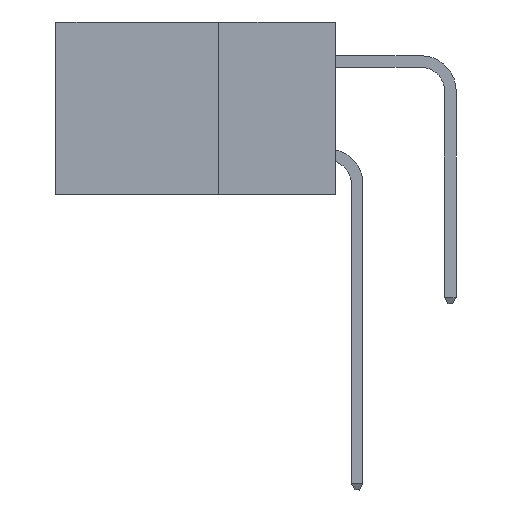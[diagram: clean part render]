
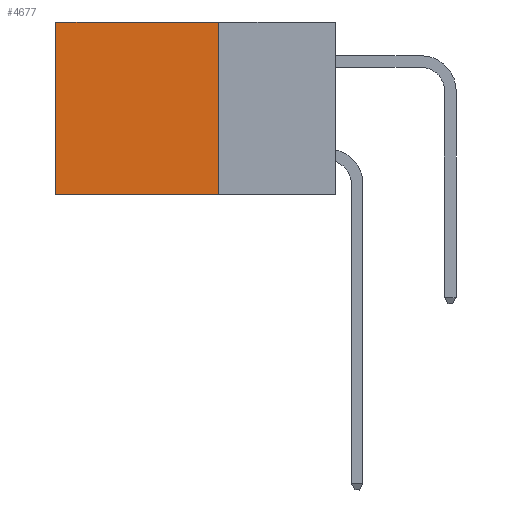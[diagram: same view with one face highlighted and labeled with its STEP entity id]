
A CAD part, left-side view. The second image highlights one B-rep face of the part: STEP entity #4677.
In plain terms, the highlighted planar face has unit normal (-1, 0, 0).
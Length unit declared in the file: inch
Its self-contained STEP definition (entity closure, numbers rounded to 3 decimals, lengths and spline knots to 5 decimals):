
#65 = DIRECTION ( 'NONE',  ( 0., 0., -1. ) ) ;
#344 = LINE ( 'NONE', #15553, #16745 ) ;
#582 = EDGE_CURVE ( 'NONE', #10924, #9720, #9602, .T. ) ;
#599 = CARTESIAN_POINT ( 'NONE',  ( 0.2875, 0.25, 0. ) ) ;
#3356 = PLANE ( 'NONE',  #12624 ) ;
#4250 = DIRECTION ( 'NONE',  ( 0., 1., 0. ) ) ;
#4677 = ADVANCED_FACE ( 'NONE', ( #23413 ), #3356, .F. ) ;
#7243 = CARTESIAN_POINT ( 'NONE',  ( 0.2875, 0.25, -0.37 ) ) ;
#8731 = DIRECTION ( 'NONE',  ( 1., 0., 0. ) ) ;
#8869 = ORIENTED_EDGE ( 'NONE', *, *, #22760, .F. ) ;
#9602 = LINE ( 'NONE', #15096, #15773 ) ;
#9717 = DIRECTION ( 'NONE',  ( 0., 1., 0. ) ) ;
#9720 = VERTEX_POINT ( 'NONE', #10195 ) ;
#10028 = ORIENTED_EDGE ( 'NONE', *, *, #582, .T. ) ;
#10195 = CARTESIAN_POINT ( 'NONE',  ( 0.2875, 0.6, 0. ) ) ;
#10525 = ORIENTED_EDGE ( 'NONE', *, *, #12679, .F. ) ;
#10576 = ORIENTED_EDGE ( 'NONE', *, *, #15108, .T. ) ;
#10594 = VECTOR ( 'NONE', #65, 39.37008 ) ;
#10787 = CARTESIAN_POINT ( 'NONE',  ( 0.2875, 0.25, 0. ) ) ;
#10924 = VERTEX_POINT ( 'NONE', #20815 ) ;
#11332 = DIRECTION ( 'NONE',  ( 0., 0., -1. ) ) ;
#12624 = AXIS2_PLACEMENT_3D ( 'NONE', #10787, #8731, #21712 ) ;
#12679 = EDGE_CURVE ( 'NONE', #10924, #15038, #20909, .T. ) ;
#13196 = CARTESIAN_POINT ( 'NONE',  ( 0.2875, 0.6, 0. ) ) ;
#13435 = LINE ( 'NONE', #13196, #10594 ) ;
#13562 = VERTEX_POINT ( 'NONE', #17308 ) ;
#15038 = VERTEX_POINT ( 'NONE', #7243 ) ;
#15096 = CARTESIAN_POINT ( 'NONE',  ( 0.2875, 0.25, 0. ) ) ;
#15108 = EDGE_CURVE ( 'NONE', #9720, #13562, #13435, .T. ) ;
#15553 = CARTESIAN_POINT ( 'NONE',  ( 0.2875, 0.25, -0.37 ) ) ;
#15773 = VECTOR ( 'NONE', #4250, 39.37008 ) ;
#16745 = VECTOR ( 'NONE', #9717, 39.37008 ) ;
#17308 = CARTESIAN_POINT ( 'NONE',  ( 0.2875, 0.6, -0.37 ) ) ;
#20815 = CARTESIAN_POINT ( 'NONE',  ( 0.2875, 0.25, 0. ) ) ;
#20909 = LINE ( 'NONE', #599, #20961 ) ;
#20961 = VECTOR ( 'NONE', #11332, 39.37008 ) ;
#21712 = DIRECTION ( 'NONE',  ( 0., 0., -1. ) ) ;
#22078 = EDGE_LOOP ( 'NONE', ( #10576, #8869, #10525, #10028 ) ) ;
#22760 = EDGE_CURVE ( 'NONE', #15038, #13562, #344, .T. ) ;
#23413 = FACE_OUTER_BOUND ( 'NONE', #22078, .T. ) ;
